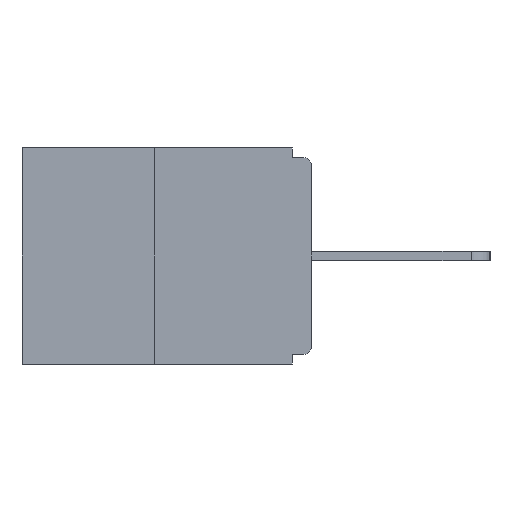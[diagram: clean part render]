
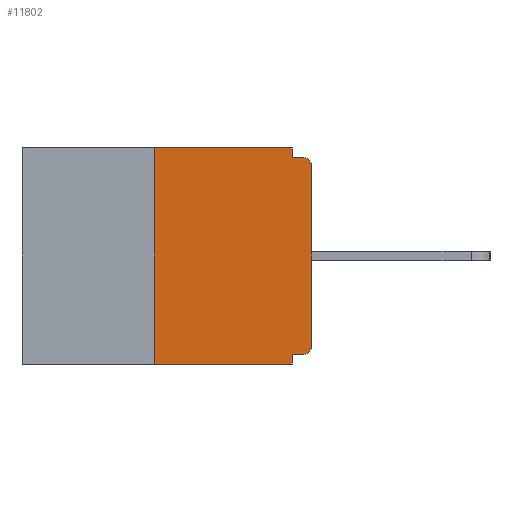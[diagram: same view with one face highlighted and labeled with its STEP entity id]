
A CAD part, left-side view. The second image highlights one B-rep face of the part: STEP entity #11802.
In plain terms, the highlighted planar face has unit normal (-1, 0, 0).
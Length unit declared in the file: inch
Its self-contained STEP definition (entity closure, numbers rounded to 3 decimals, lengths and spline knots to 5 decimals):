
#17 = VECTOR ( 'NONE', #679, 39.37008 ) ;
#97 = CARTESIAN_POINT ( 'NONE',  ( 0., 0.46, 0. ) ) ;
#494 = LINE ( 'NONE', #2940, #13023 ) ;
#581 = LINE ( 'NONE', #10788, #7462 ) ;
#679 = DIRECTION ( 'NONE',  ( 0., 0., -1. ) ) ;
#875 = CARTESIAN_POINT ( 'NONE',  ( 0., 0.25, -0.343 ) ) ;
#896 = ORIENTED_EDGE ( 'NONE', *, *, #10562, .F. ) ;
#971 = LINE ( 'NONE', #14163, #13705 ) ;
#1378 = EDGE_CURVE ( 'NONE', #10367, #16763, #16072, .T. ) ;
#1422 = DIRECTION ( 'NONE',  ( 0., 0., 1. ) ) ;
#1452 = CIRCLE ( 'NONE', #14844, 0.015 ) ;
#1809 = FACE_OUTER_BOUND ( 'NONE', #10440, .T. ) ;
#1931 = DIRECTION ( 'NONE',  ( 0., 1., 0. ) ) ;
#1967 = VECTOR ( 'NONE', #12718, 39.37008 ) ;
#2066 = CARTESIAN_POINT ( 'NONE',  ( 0., 0.46, 0. ) ) ;
#2237 = CARTESIAN_POINT ( 'NONE',  ( 0., 0., -0.03 ) ) ;
#2336 = LINE ( 'NONE', #10176, #8553 ) ;
#2419 = CARTESIAN_POINT ( 'NONE',  ( 0., 0., -0.313 ) ) ;
#2704 = DIRECTION ( 'NONE',  ( 0., 0., -1. ) ) ;
#2773 = DIRECTION ( 'NONE',  ( 0., -1., 0. ) ) ;
#2940 = CARTESIAN_POINT ( 'NONE',  ( 0., 0.46, -0.343 ) ) ;
#3031 = DIRECTION ( 'NONE',  ( 0., -1., 0. ) ) ;
#3050 = AXIS2_PLACEMENT_3D ( 'NONE', #97, #5302, #2704 ) ;
#3064 = CARTESIAN_POINT ( 'NONE',  ( 0., 0.25, 0. ) ) ;
#3624 = VERTEX_POINT ( 'NONE', #6760 ) ;
#4310 = DIRECTION ( 'NONE',  ( 0., 0., -1. ) ) ;
#4352 = EDGE_CURVE ( 'NONE', #3624, #10367, #9660, .T. ) ;
#4356 = AXIS2_PLACEMENT_3D ( 'NONE', #8426, #13933, #4310 ) ;
#4580 = CARTESIAN_POINT ( 'NONE',  ( 0., 0.031, -0.328 ) ) ;
#5302 = DIRECTION ( 'NONE',  ( 1., 0., 0. ) ) ;
#5854 = ORIENTED_EDGE ( 'NONE', *, *, #15051, .T. ) ;
#5921 = DIRECTION ( 'NONE',  ( -1., 0., 0. ) ) ;
#6103 = ORIENTED_EDGE ( 'NONE', *, *, #12580, .F. ) ;
#6237 = DIRECTION ( 'NONE',  ( 0., 0., -1. ) ) ;
#6257 = VECTOR ( 'NONE', #1422, 39.37008 ) ;
#6617 = PLANE ( 'NONE',  #3050 ) ;
#6671 = ORIENTED_EDGE ( 'NONE', *, *, #15041, .F. ) ;
#6760 = CARTESIAN_POINT ( 'NONE',  ( 0., 0.015, -0.328 ) ) ;
#6952 = CARTESIAN_POINT ( 'NONE',  ( 0., 0., -0.015 ) ) ;
#7027 = VERTEX_POINT ( 'NONE', #14376 ) ;
#7040 = VECTOR ( 'NONE', #3031, 39.37008 ) ;
#7462 = VECTOR ( 'NONE', #14846, 39.37008 ) ;
#7583 = CARTESIAN_POINT ( 'NONE',  ( 0., 0.031, -0.343 ) ) ;
#8426 = CARTESIAN_POINT ( 'NONE',  ( 0., 0.015, -0.313 ) ) ;
#8429 = VERTEX_POINT ( 'NONE', #3064 ) ;
#8450 = LINE ( 'NONE', #15108, #17 ) ;
#8553 = VECTOR ( 'NONE', #6237, 39.37008 ) ;
#9011 = EDGE_CURVE ( 'NONE', #10665, #13574, #2336, .T. ) ;
#9240 = ORIENTED_EDGE ( 'NONE', *, *, #9268, .T. ) ;
#9268 = EDGE_CURVE ( 'NONE', #12375, #13574, #494, .T. ) ;
#9660 = CIRCLE ( 'NONE', #4356, 0.015 ) ;
#9662 = LINE ( 'NONE', #6952, #7040 ) ;
#10176 = CARTESIAN_POINT ( 'NONE',  ( 0., 0.031, -0.343 ) ) ;
#10367 = VERTEX_POINT ( 'NONE', #2419 ) ;
#10440 = EDGE_LOOP ( 'NONE', ( #15714, #896, #9240, #16451, #6671, #14911, #14571, #5854, #11323, #6103 ) ) ;
#10562 = EDGE_CURVE ( 'NONE', #12375, #8429, #581, .T. ) ;
#10665 = VERTEX_POINT ( 'NONE', #4580 ) ;
#10788 = CARTESIAN_POINT ( 'NONE',  ( 0., 0.25, 0. ) ) ;
#11323 = ORIENTED_EDGE ( 'NONE', *, *, #16519, .F. ) ;
#11514 = DIRECTION ( 'NONE',  ( 0., 0., -1. ) ) ;
#11802 = ADVANCED_FACE ( 'NONE', ( #1809 ), #6617, .F. ) ;
#12055 = CARTESIAN_POINT ( 'NONE',  ( 0., 0., 0. ) ) ;
#12079 = VERTEX_POINT ( 'NONE', #15860 ) ;
#12263 = CARTESIAN_POINT ( 'NONE',  ( 0., 0.031, -0.015 ) ) ;
#12375 = VERTEX_POINT ( 'NONE', #875 ) ;
#12580 = EDGE_CURVE ( 'NONE', #12079, #17025, #8450, .T. ) ;
#12718 = DIRECTION ( 'NONE',  ( 0., -1., 0. ) ) ;
#12817 = EDGE_CURVE ( 'NONE', #8429, #12079, #14043, .T. ) ;
#13023 = VECTOR ( 'NONE', #2773, 39.37008 ) ;
#13574 = VERTEX_POINT ( 'NONE', #7583 ) ;
#13705 = VECTOR ( 'NONE', #1931, 39.37008 ) ;
#13933 = DIRECTION ( 'NONE',  ( -1., 0., 0. ) ) ;
#14043 = LINE ( 'NONE', #2066, #1967 ) ;
#14163 = CARTESIAN_POINT ( 'NONE',  ( 0., 0., -0.328 ) ) ;
#14376 = CARTESIAN_POINT ( 'NONE',  ( 0., 0.015, -0.015 ) ) ;
#14571 = ORIENTED_EDGE ( 'NONE', *, *, #1378, .T. ) ;
#14844 = AXIS2_PLACEMENT_3D ( 'NONE', #16597, #5921, #11514 ) ;
#14846 = DIRECTION ( 'NONE',  ( 0., 0., 1. ) ) ;
#14911 = ORIENTED_EDGE ( 'NONE', *, *, #4352, .T. ) ;
#15041 = EDGE_CURVE ( 'NONE', #3624, #10665, #971, .T. ) ;
#15051 = EDGE_CURVE ( 'NONE', #16763, #7027, #1452, .T. ) ;
#15108 = CARTESIAN_POINT ( 'NONE',  ( 0., 0.031, 0. ) ) ;
#15714 = ORIENTED_EDGE ( 'NONE', *, *, #12817, .F. ) ;
#15860 = CARTESIAN_POINT ( 'NONE',  ( 0., 0.031, 0. ) ) ;
#16072 = LINE ( 'NONE', #12055, #6257 ) ;
#16451 = ORIENTED_EDGE ( 'NONE', *, *, #9011, .F. ) ;
#16519 = EDGE_CURVE ( 'NONE', #17025, #7027, #9662, .T. ) ;
#16597 = CARTESIAN_POINT ( 'NONE',  ( 0., 0.015, -0.03 ) ) ;
#16763 = VERTEX_POINT ( 'NONE', #2237 ) ;
#17025 = VERTEX_POINT ( 'NONE', #12263 ) ;
